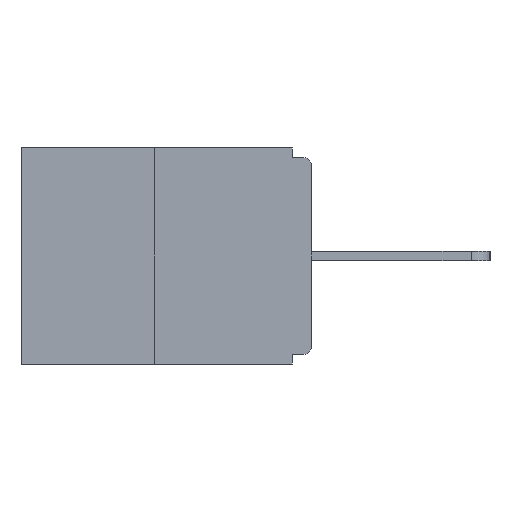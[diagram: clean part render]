
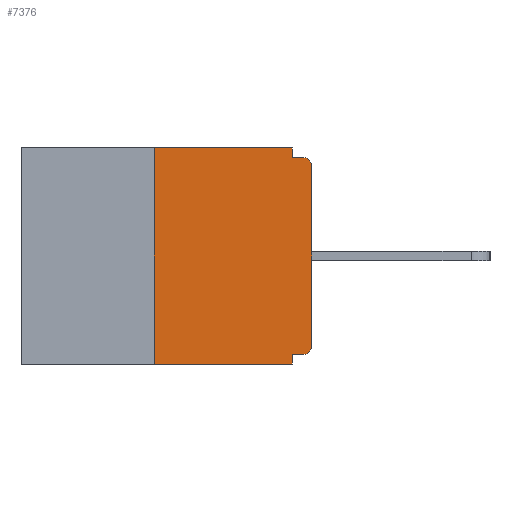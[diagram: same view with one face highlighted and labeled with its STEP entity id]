
A CAD part, left-side view. The second image highlights one B-rep face of the part: STEP entity #7376.
In plain terms, the highlighted planar face has unit normal (-1, 0, 0).
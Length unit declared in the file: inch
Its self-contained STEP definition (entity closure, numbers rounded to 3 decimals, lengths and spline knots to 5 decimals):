
#238 = CIRCLE ( 'NONE', #4943, 0.015 ) ;
#310 = EDGE_CURVE ( 'NONE', #7810, #2796, #7860, .T. ) ;
#440 = LINE ( 'NONE', #9470, #8924 ) ;
#986 = DIRECTION ( 'NONE',  ( 0., 0., 1. ) ) ;
#1708 = ORIENTED_EDGE ( 'NONE', *, *, #4015, .F. ) ;
#1723 = DIRECTION ( 'NONE',  ( 0., -1., 0. ) ) ;
#1764 = CARTESIAN_POINT ( 'NONE',  ( 0., 0.031, -0.343 ) ) ;
#2247 = DIRECTION ( 'NONE',  ( 1., 0., 0. ) ) ;
#2286 = EDGE_CURVE ( 'NONE', #9834, #7231, #9596, .T. ) ;
#2356 = CARTESIAN_POINT ( 'NONE',  ( 0., 0.46, 0. ) ) ;
#2431 = DIRECTION ( 'NONE',  ( 0., 0., -1. ) ) ;
#2465 = DIRECTION ( 'NONE',  ( 0., 0., 1. ) ) ;
#2487 = DIRECTION ( 'NONE',  ( -1., 0., 0. ) ) ;
#2540 = DIRECTION ( 'NONE',  ( 0., 0., -1. ) ) ;
#2610 = DIRECTION ( 'NONE',  ( 0., 0., -1. ) ) ;
#2670 = CARTESIAN_POINT ( 'NONE',  ( 0., 0.015, -0.015 ) ) ;
#2796 = VERTEX_POINT ( 'NONE', #1764 ) ;
#2800 = ORIENTED_EDGE ( 'NONE', *, *, #11494, .T. ) ;
#2835 = DIRECTION ( 'NONE',  ( 0., -1., 0. ) ) ;
#2921 = DIRECTION ( 'NONE',  ( 0., -1., 0. ) ) ;
#2989 = ORIENTED_EDGE ( 'NONE', *, *, #4640, .F. ) ;
#3128 = EDGE_CURVE ( 'NONE', #5054, #2796, #7945, .T. ) ;
#4015 = EDGE_CURVE ( 'NONE', #9446, #8384, #10959, .T. ) ;
#4047 = DIRECTION ( 'NONE',  ( 0., 0., -1. ) ) ;
#4106 = VECTOR ( 'NONE', #1723, 39.37008 ) ;
#4366 = ORIENTED_EDGE ( 'NONE', *, *, #310, .F. ) ;
#4492 = AXIS2_PLACEMENT_3D ( 'NONE', #8697, #2487, #2431 ) ;
#4567 = LINE ( 'NONE', #8898, #6007 ) ;
#4640 = EDGE_CURVE ( 'NONE', #9834, #7810, #6440, .T. ) ;
#4893 = CARTESIAN_POINT ( 'NONE',  ( 0., 0., 0. ) ) ;
#4943 = AXIS2_PLACEMENT_3D ( 'NONE', #5205, #7041, #2610 ) ;
#5009 = EDGE_CURVE ( 'NONE', #5054, #5197, #4567, .T. ) ;
#5054 = VERTEX_POINT ( 'NONE', #9844 ) ;
#5197 = VERTEX_POINT ( 'NONE', #8532 ) ;
#5205 = CARTESIAN_POINT ( 'NONE',  ( 0., 0.015, -0.03 ) ) ;
#5265 = CARTESIAN_POINT ( 'NONE',  ( 0., 0.031, 0. ) ) ;
#5426 = VECTOR ( 'NONE', #6496, 39.37008 ) ;
#5856 = DIRECTION ( 'NONE',  ( 0., 0., -1. ) ) ;
#6007 = VECTOR ( 'NONE', #986, 39.37008 ) ;
#6022 = CARTESIAN_POINT ( 'NONE',  ( 0., 0.031, -0.328 ) ) ;
#6027 = ORIENTED_EDGE ( 'NONE', *, *, #3128, .T. ) ;
#6165 = ORIENTED_EDGE ( 'NONE', *, *, #2286, .T. ) ;
#6218 = CARTESIAN_POINT ( 'NONE',  ( 0., 0.031, -0.343 ) ) ;
#6302 = VECTOR ( 'NONE', #2540, 39.37008 ) ;
#6384 = CARTESIAN_POINT ( 'NONE',  ( 0., 0., -0.328 ) ) ;
#6440 = LINE ( 'NONE', #6384, #5426 ) ;
#6496 = DIRECTION ( 'NONE',  ( 0., 1., 0. ) ) ;
#6798 = FACE_OUTER_BOUND ( 'NONE', #7253, .T. ) ;
#7041 = DIRECTION ( 'NONE',  ( -1., 0., 0. ) ) ;
#7154 = CARTESIAN_POINT ( 'NONE',  ( 0., 0., -0.015 ) ) ;
#7231 = VERTEX_POINT ( 'NONE', #11092 ) ;
#7253 = EDGE_LOOP ( 'NONE', ( #11310, #8657, #6027, #4366, #2989, #6165, #9898, #2800, #1708, #10757 ) ) ;
#7376 = ADVANCED_FACE ( 'NONE', ( #6798 ), #10553, .F. ) ;
#7760 = EDGE_CURVE ( 'NONE', #7231, #8480, #7842, .T. ) ;
#7810 = VERTEX_POINT ( 'NONE', #6022 ) ;
#7842 = LINE ( 'NONE', #4893, #10317 ) ;
#7860 = LINE ( 'NONE', #6218, #6302 ) ;
#7945 = LINE ( 'NONE', #10059, #11039 ) ;
#8052 = CARTESIAN_POINT ( 'NONE',  ( 0., 0., -0.03 ) ) ;
#8370 = EDGE_CURVE ( 'NONE', #5197, #8895, #10798, .T. ) ;
#8384 = VERTEX_POINT ( 'NONE', #2670 ) ;
#8403 = CARTESIAN_POINT ( 'NONE',  ( 0., 0.015, -0.328 ) ) ;
#8480 = VERTEX_POINT ( 'NONE', #8052 ) ;
#8532 = CARTESIAN_POINT ( 'NONE',  ( 0., 0.25, 0. ) ) ;
#8657 = ORIENTED_EDGE ( 'NONE', *, *, #5009, .F. ) ;
#8697 = CARTESIAN_POINT ( 'NONE',  ( 0., 0.015, -0.313 ) ) ;
#8895 = VERTEX_POINT ( 'NONE', #5265 ) ;
#8898 = CARTESIAN_POINT ( 'NONE',  ( 0., 0.25, 0. ) ) ;
#8924 = VECTOR ( 'NONE', #4047, 39.37008 ) ;
#8996 = VECTOR ( 'NONE', #2835, 39.37008 ) ;
#9446 = VERTEX_POINT ( 'NONE', #11059 ) ;
#9470 = CARTESIAN_POINT ( 'NONE',  ( 0., 0.031, 0. ) ) ;
#9596 = CIRCLE ( 'NONE', #4492, 0.015 ) ;
#9634 = EDGE_CURVE ( 'NONE', #8895, #9446, #440, .T. ) ;
#9821 = CARTESIAN_POINT ( 'NONE',  ( 0., 0.46, 0. ) ) ;
#9834 = VERTEX_POINT ( 'NONE', #8403 ) ;
#9844 = CARTESIAN_POINT ( 'NONE',  ( 0., 0.25, -0.343 ) ) ;
#9898 = ORIENTED_EDGE ( 'NONE', *, *, #7760, .T. ) ;
#10059 = CARTESIAN_POINT ( 'NONE',  ( 0., 0.46, -0.343 ) ) ;
#10309 = AXIS2_PLACEMENT_3D ( 'NONE', #2356, #2247, #5856 ) ;
#10317 = VECTOR ( 'NONE', #2465, 39.37008 ) ;
#10553 = PLANE ( 'NONE',  #10309 ) ;
#10757 = ORIENTED_EDGE ( 'NONE', *, *, #9634, .F. ) ;
#10798 = LINE ( 'NONE', #9821, #4106 ) ;
#10959 = LINE ( 'NONE', #7154, #8996 ) ;
#11039 = VECTOR ( 'NONE', #2921, 39.37008 ) ;
#11059 = CARTESIAN_POINT ( 'NONE',  ( 0., 0.031, -0.015 ) ) ;
#11092 = CARTESIAN_POINT ( 'NONE',  ( 0., 0., -0.313 ) ) ;
#11310 = ORIENTED_EDGE ( 'NONE', *, *, #8370, .F. ) ;
#11494 = EDGE_CURVE ( 'NONE', #8480, #8384, #238, .T. ) ;
